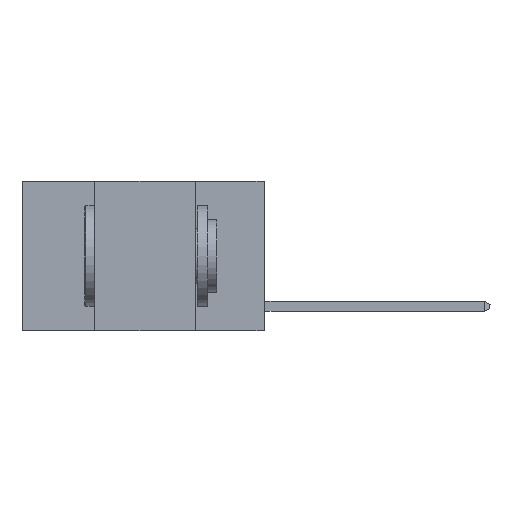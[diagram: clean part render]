
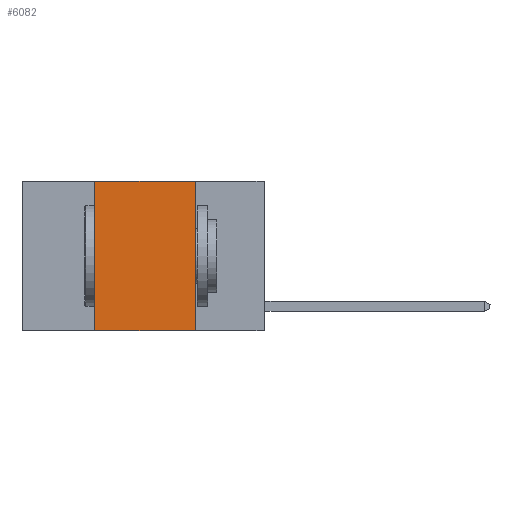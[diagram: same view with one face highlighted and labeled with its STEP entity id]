
A CAD part, left-side view. The second image highlights one B-rep face of the part: STEP entity #6082.
In plain terms, the highlighted planar face has unit normal (-1, 0, 0).
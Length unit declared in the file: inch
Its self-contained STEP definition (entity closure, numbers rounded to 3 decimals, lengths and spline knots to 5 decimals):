
#554 = DIRECTION ( 'NONE',  ( 1., 0., 0. ) ) ;
#1177 = LINE ( 'NONE', #4853, #16545 ) ;
#1411 = CARTESIAN_POINT ( 'NONE',  ( 0., 0.42, 0. ) ) ;
#1571 = ORIENTED_EDGE ( 'NONE', *, *, #18196, .T. ) ;
#1918 = VECTOR ( 'NONE', #19571, 39.37008 ) ;
#2678 = VERTEX_POINT ( 'NONE', #7354 ) ;
#3013 = DIRECTION ( 'NONE',  ( 0., 0., -1. ) ) ;
#4375 = PLANE ( 'NONE',  #7513 ) ;
#4853 = CARTESIAN_POINT ( 'NONE',  ( 0., 0.17, 0. ) ) ;
#5222 = EDGE_CURVE ( 'NONE', #19199, #23123, #12853, .T. ) ;
#5251 = EDGE_CURVE ( 'NONE', #2678, #21157, #1177, .T. ) ;
#5504 = CARTESIAN_POINT ( 'NONE',  ( 0., 0.6, -0.37 ) ) ;
#6082 = ADVANCED_FACE ( 'NONE', ( #14115 ), #4375, .F. ) ;
#6651 = LINE ( 'NONE', #16287, #16965 ) ;
#7354 = CARTESIAN_POINT ( 'NONE',  ( 0., 0.17, 0. ) ) ;
#7487 = CARTESIAN_POINT ( 'NONE',  ( 0., 0.42, -0.37 ) ) ;
#7513 = AXIS2_PLACEMENT_3D ( 'NONE', #19811, #554, #8043 ) ;
#8043 = DIRECTION ( 'NONE',  ( 0., 0., -1. ) ) ;
#8152 = LINE ( 'NONE', #5504, #1918 ) ;
#9575 = CARTESIAN_POINT ( 'NONE',  ( 0., 0.42, 0. ) ) ;
#9764 = CARTESIAN_POINT ( 'NONE',  ( 0., 0.17, -0.37 ) ) ;
#10619 = DIRECTION ( 'NONE',  ( 0., 0., 1. ) ) ;
#12362 = ORIENTED_EDGE ( 'NONE', *, *, #5222, .F. ) ;
#12853 = LINE ( 'NONE', #1411, #13357 ) ;
#12975 = ORIENTED_EDGE ( 'NONE', *, *, #5251, .F. ) ;
#13357 = VECTOR ( 'NONE', #10619, 39.37008 ) ;
#14115 = FACE_OUTER_BOUND ( 'NONE', #20956, .T. ) ;
#15021 = ORIENTED_EDGE ( 'NONE', *, *, #19964, .F. ) ;
#16287 = CARTESIAN_POINT ( 'NONE',  ( 0., 0.6, 0. ) ) ;
#16545 = VECTOR ( 'NONE', #3013, 39.37008 ) ;
#16965 = VECTOR ( 'NONE', #21989, 39.37008 ) ;
#18196 = EDGE_CURVE ( 'NONE', #19199, #21157, #8152, .T. ) ;
#19199 = VERTEX_POINT ( 'NONE', #7487 ) ;
#19571 = DIRECTION ( 'NONE',  ( 0., -1., 0. ) ) ;
#19811 = CARTESIAN_POINT ( 'NONE',  ( 0., 0.6, 0. ) ) ;
#19964 = EDGE_CURVE ( 'NONE', #23123, #2678, #6651, .T. ) ;
#20956 = EDGE_LOOP ( 'NONE', ( #12975, #15021, #12362, #1571 ) ) ;
#21157 = VERTEX_POINT ( 'NONE', #9764 ) ;
#21989 = DIRECTION ( 'NONE',  ( 0., -1., 0. ) ) ;
#23123 = VERTEX_POINT ( 'NONE', #9575 ) ;
